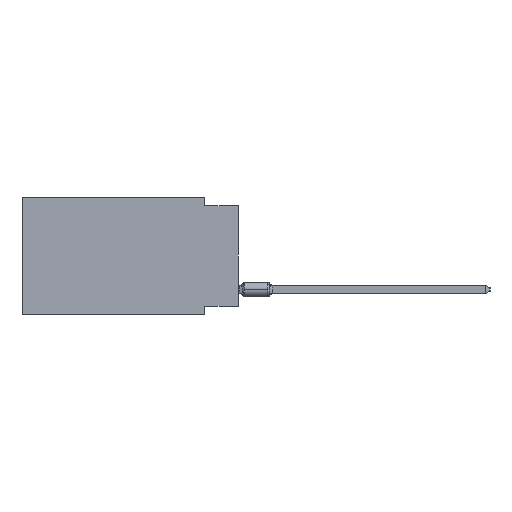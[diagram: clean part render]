
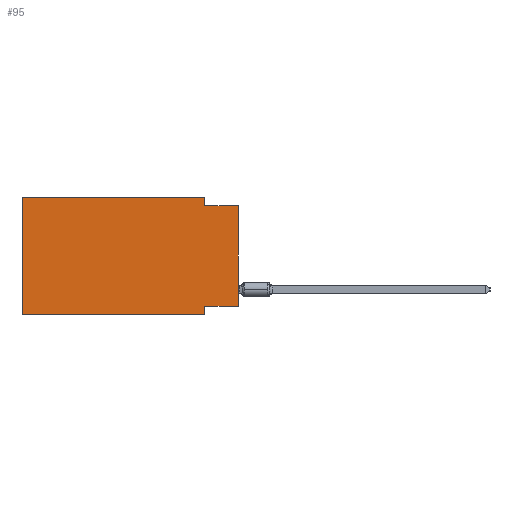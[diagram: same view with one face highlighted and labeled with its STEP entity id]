
A CAD part, left-side view. The second image highlights one B-rep face of the part: STEP entity #95.
In plain terms, the highlighted planar face has unit normal (-1, 0, 0).
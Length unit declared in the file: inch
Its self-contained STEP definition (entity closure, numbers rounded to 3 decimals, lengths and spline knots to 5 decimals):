
#95 = ADVANCED_FACE ( 'NONE', ( #10595 ), #12738, .F. ) ;
#164 = DIRECTION ( 'NONE',  ( 0., 0., -1. ) ) ;
#358 = LINE ( 'NONE', #6992, #7134 ) ;
#943 = ORIENTED_EDGE ( 'NONE', *, *, #1424, .F. ) ;
#1338 = VECTOR ( 'NONE', #164, 39.37008 ) ;
#1424 = EDGE_CURVE ( 'NONE', #22831, #13278, #11769, .T. ) ;
#1838 = EDGE_CURVE ( 'NONE', #16454, #14864, #14652, .T. ) ;
#2364 = CARTESIAN_POINT ( 'NONE',  ( 0., 0.1, -0.35 ) ) ;
#2392 = VECTOR ( 'NONE', #27987, 39.37008 ) ;
#2956 = CARTESIAN_POINT ( 'NONE',  ( 0., 0.1, 0. ) ) ;
#3821 = DIRECTION ( 'NONE',  ( 0., 0., -1. ) ) ;
#3940 = VECTOR ( 'NONE', #9613, 39.37008 ) ;
#4575 = ORIENTED_EDGE ( 'NONE', *, *, #8818, .F. ) ;
#5810 = CARTESIAN_POINT ( 'NONE',  ( 0., 0., -0.025 ) ) ;
#6035 = CARTESIAN_POINT ( 'NONE',  ( 0., 0.1, -0.025 ) ) ;
#6074 = VECTOR ( 'NONE', #7640, 39.37008 ) ;
#6584 = CARTESIAN_POINT ( 'NONE',  ( 0., 0., 0. ) ) ;
#6818 = DIRECTION ( 'NONE',  ( 0., -1., 0. ) ) ;
#6992 = CARTESIAN_POINT ( 'NONE',  ( 0., 0.645, -0.35 ) ) ;
#7134 = VECTOR ( 'NONE', #28250, 39.37008 ) ;
#7341 = CARTESIAN_POINT ( 'NONE',  ( 0., 0.645, -0.35 ) ) ;
#7497 = VECTOR ( 'NONE', #6818, 39.37008 ) ;
#7640 = DIRECTION ( 'NONE',  ( 0., 0., 1. ) ) ;
#7746 = CARTESIAN_POINT ( 'NONE',  ( 0., 0.645, 0. ) ) ;
#7955 = LINE ( 'NONE', #19503, #30194 ) ;
#8818 = EDGE_CURVE ( 'NONE', #28137, #22831, #7955, .T. ) ;
#8995 = EDGE_CURVE ( 'NONE', #14864, #18827, #10735, .T. ) ;
#9613 = DIRECTION ( 'NONE',  ( 0., 0., -1. ) ) ;
#10595 = FACE_OUTER_BOUND ( 'NONE', #14120, .T. ) ;
#10735 = LINE ( 'NONE', #5810, #7497 ) ;
#10945 = VERTEX_POINT ( 'NONE', #7746 ) ;
#11769 = LINE ( 'NONE', #2364, #3940 ) ;
#12738 = PLANE ( 'NONE',  #28884 ) ;
#12992 = ORIENTED_EDGE ( 'NONE', *, *, #15809, .F. ) ;
#13227 = EDGE_CURVE ( 'NONE', #10945, #16454, #14511, .T. ) ;
#13278 = VERTEX_POINT ( 'NONE', #20989 ) ;
#14120 = EDGE_LOOP ( 'NONE', ( #15281, #26958, #29489, #18862, #12992, #18577, #943, #4575 ) ) ;
#14244 = CARTESIAN_POINT ( 'NONE',  ( 0., 0.645, 0. ) ) ;
#14511 = LINE ( 'NONE', #23608, #25748 ) ;
#14571 = DIRECTION ( 'NONE',  ( 0., 1., 0. ) ) ;
#14652 = LINE ( 'NONE', #2956, #1338 ) ;
#14785 = EDGE_CURVE ( 'NONE', #19215, #13278, #358, .T. ) ;
#14864 = VERTEX_POINT ( 'NONE', #6035 ) ;
#15281 = ORIENTED_EDGE ( 'NONE', *, *, #19063, .T. ) ;
#15809 = EDGE_CURVE ( 'NONE', #19215, #10945, #23809, .T. ) ;
#16454 = VERTEX_POINT ( 'NONE', #27156 ) ;
#18362 = CARTESIAN_POINT ( 'NONE',  ( 0., 0., -0.325 ) ) ;
#18577 = ORIENTED_EDGE ( 'NONE', *, *, #14785, .T. ) ;
#18578 = LINE ( 'NONE', #6584, #2392 ) ;
#18827 = VERTEX_POINT ( 'NONE', #21230 ) ;
#18862 = ORIENTED_EDGE ( 'NONE', *, *, #13227, .F. ) ;
#19063 = EDGE_CURVE ( 'NONE', #28137, #18827, #18578, .T. ) ;
#19215 = VERTEX_POINT ( 'NONE', #7341 ) ;
#19503 = CARTESIAN_POINT ( 'NONE',  ( 0., 0., -0.325 ) ) ;
#20989 = CARTESIAN_POINT ( 'NONE',  ( 0., 0.1, -0.35 ) ) ;
#21230 = CARTESIAN_POINT ( 'NONE',  ( 0., 0., -0.025 ) ) ;
#22138 = CARTESIAN_POINT ( 'NONE',  ( 0., 0.645, 0. ) ) ;
#22831 = VERTEX_POINT ( 'NONE', #25865 ) ;
#23608 = CARTESIAN_POINT ( 'NONE',  ( 0., 0.645, 0. ) ) ;
#23809 = LINE ( 'NONE', #14244, #6074 ) ;
#25748 = VECTOR ( 'NONE', #28234, 39.37008 ) ;
#25865 = CARTESIAN_POINT ( 'NONE',  ( 0., 0.1, -0.325 ) ) ;
#26958 = ORIENTED_EDGE ( 'NONE', *, *, #8995, .F. ) ;
#27156 = CARTESIAN_POINT ( 'NONE',  ( 0., 0.1, 0. ) ) ;
#27987 = DIRECTION ( 'NONE',  ( 0., 0., 1. ) ) ;
#28137 = VERTEX_POINT ( 'NONE', #18362 ) ;
#28234 = DIRECTION ( 'NONE',  ( 0., -1., 0. ) ) ;
#28250 = DIRECTION ( 'NONE',  ( 0., -1., 0. ) ) ;
#28884 = AXIS2_PLACEMENT_3D ( 'NONE', #22138, #29225, #3821 ) ;
#29225 = DIRECTION ( 'NONE',  ( 1., 0., 0. ) ) ;
#29489 = ORIENTED_EDGE ( 'NONE', *, *, #1838, .F. ) ;
#30194 = VECTOR ( 'NONE', #14571, 39.37008 ) ;
